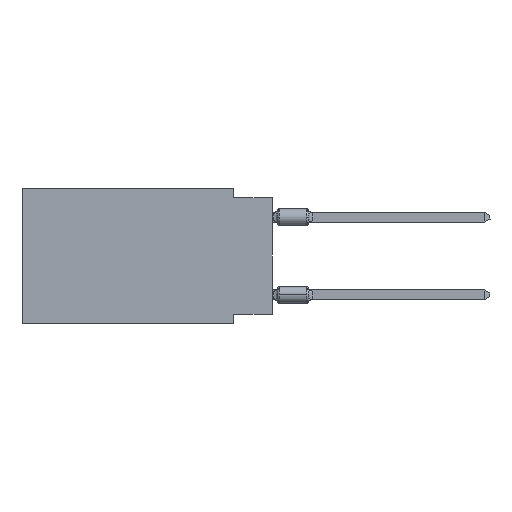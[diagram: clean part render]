
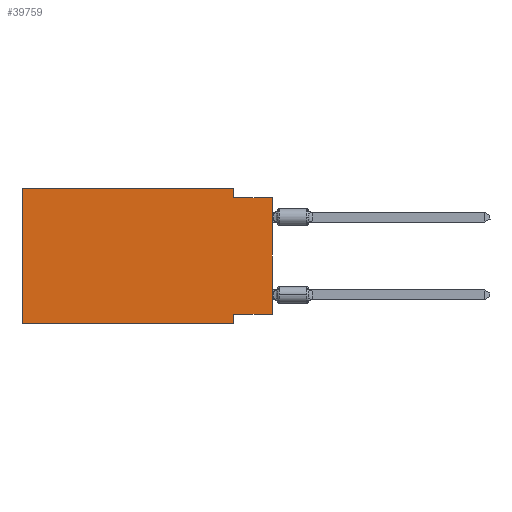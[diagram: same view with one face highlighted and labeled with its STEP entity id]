
A CAD part, left-side view. The second image highlights one B-rep face of the part: STEP entity #39759.
In plain terms, the highlighted planar face has unit normal (-1, 0, 0).
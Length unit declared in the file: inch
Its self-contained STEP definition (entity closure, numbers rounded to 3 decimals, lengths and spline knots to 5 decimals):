
#1094 = EDGE_CURVE ( 'NONE', #7200, #34271, #24321, .T. ) ;
#1792 = DIRECTION ( 'NONE',  ( 0., -1., 0. ) ) ;
#2064 = VECTOR ( 'NONE', #16429, 39.37008 ) ;
#2184 = DIRECTION ( 'NONE',  ( 0., 0., -1. ) ) ;
#2597 = DIRECTION ( 'NONE',  ( 0., 0., -1. ) ) ;
#3009 = VERTEX_POINT ( 'NONE', #53379 ) ;
#3027 = CARTESIAN_POINT ( 'NONE',  ( 0., 0.645, -0.35 ) ) ;
#5474 = CARTESIAN_POINT ( 'NONE',  ( 0., 0.1, -0.325 ) ) ;
#5514 = CARTESIAN_POINT ( 'NONE',  ( 0., 0.1, -0.025 ) ) ;
#6028 = CARTESIAN_POINT ( 'NONE',  ( 0., 0.645, 0. ) ) ;
#6404 = EDGE_CURVE ( 'NONE', #3009, #37174, #39988, .T. ) ;
#6475 = DIRECTION ( 'NONE',  ( 0., 1., 0. ) ) ;
#6872 = ORIENTED_EDGE ( 'NONE', *, *, #6404, .F. ) ;
#7200 = VERTEX_POINT ( 'NONE', #22787 ) ;
#7378 = EDGE_CURVE ( 'NONE', #37174, #37012, #45947, .T. ) ;
#9947 = LINE ( 'NONE', #36362, #50279 ) ;
#12422 = ORIENTED_EDGE ( 'NONE', *, *, #31131, .T. ) ;
#13573 = CARTESIAN_POINT ( 'NONE',  ( 0., 0.645, 0. ) ) ;
#15375 = AXIS2_PLACEMENT_3D ( 'NONE', #69291, #51464, #2597 ) ;
#16429 = DIRECTION ( 'NONE',  ( 0., 0., 1. ) ) ;
#19960 = DIRECTION ( 'NONE',  ( 0., -1., 0. ) ) ;
#20821 = ORIENTED_EDGE ( 'NONE', *, *, #7378, .F. ) ;
#22787 = CARTESIAN_POINT ( 'NONE',  ( 0., 0., -0.325 ) ) ;
#23121 = CARTESIAN_POINT ( 'NONE',  ( 0., 0.1, -0.35 ) ) ;
#23978 = CARTESIAN_POINT ( 'NONE',  ( 0., 0., -0.325 ) ) ;
#24211 = LINE ( 'NONE', #61638, #42753 ) ;
#24321 = LINE ( 'NONE', #23978, #45250 ) ;
#24451 = ORIENTED_EDGE ( 'NONE', *, *, #54711, .T. ) ;
#25794 = PLANE ( 'NONE',  #15375 ) ;
#27500 = DIRECTION ( 'NONE',  ( 0., 0., 1. ) ) ;
#27791 = CARTESIAN_POINT ( 'NONE',  ( 0., 0., -0.025 ) ) ;
#27834 = EDGE_CURVE ( 'NONE', #51029, #43485, #70277, .T. ) ;
#29914 = DIRECTION ( 'NONE',  ( 0., 0., -1. ) ) ;
#31131 = EDGE_CURVE ( 'NONE', #51029, #47694, #9947, .T. ) ;
#34271 = VERTEX_POINT ( 'NONE', #5474 ) ;
#36362 = CARTESIAN_POINT ( 'NONE',  ( 0., 0.645, -0.35 ) ) ;
#37012 = VERTEX_POINT ( 'NONE', #27791 ) ;
#37174 = VERTEX_POINT ( 'NONE', #5514 ) ;
#39305 = ORIENTED_EDGE ( 'NONE', *, *, #27834, .F. ) ;
#39759 = ADVANCED_FACE ( 'NONE', ( #52894 ), #25794, .F. ) ;
#39988 = LINE ( 'NONE', #55375, #59538 ) ;
#40474 = EDGE_CURVE ( 'NONE', #34271, #47694, #24211, .T. ) ;
#41664 = CARTESIAN_POINT ( 'NONE',  ( 0., 0., -0.025 ) ) ;
#42728 = EDGE_CURVE ( 'NONE', #43485, #3009, #62416, .T. ) ;
#42753 = VECTOR ( 'NONE', #29914, 39.37008 ) ;
#43485 = VERTEX_POINT ( 'NONE', #53410 ) ;
#45250 = VECTOR ( 'NONE', #6475, 39.37008 ) ;
#45718 = VECTOR ( 'NONE', #1792, 39.37008 ) ;
#45947 = LINE ( 'NONE', #41664, #47339 ) ;
#46823 = VECTOR ( 'NONE', #27500, 39.37008 ) ;
#47339 = VECTOR ( 'NONE', #68039, 39.37008 ) ;
#47694 = VERTEX_POINT ( 'NONE', #23121 ) ;
#50279 = VECTOR ( 'NONE', #19960, 39.37008 ) ;
#51029 = VERTEX_POINT ( 'NONE', #3027 ) ;
#51464 = DIRECTION ( 'NONE',  ( 1., 0., 0. ) ) ;
#52894 = FACE_OUTER_BOUND ( 'NONE', #61762, .T. ) ;
#53379 = CARTESIAN_POINT ( 'NONE',  ( 0., 0.1, 0. ) ) ;
#53410 = CARTESIAN_POINT ( 'NONE',  ( 0., 0.645, 0. ) ) ;
#54711 = EDGE_CURVE ( 'NONE', #7200, #37012, #65986, .T. ) ;
#54886 = ORIENTED_EDGE ( 'NONE', *, *, #1094, .F. ) ;
#55375 = CARTESIAN_POINT ( 'NONE',  ( 0., 0.1, 0. ) ) ;
#59538 = VECTOR ( 'NONE', #2184, 39.37008 ) ;
#59875 = ORIENTED_EDGE ( 'NONE', *, *, #40474, .F. ) ;
#61638 = CARTESIAN_POINT ( 'NONE',  ( 0., 0.1, -0.35 ) ) ;
#61762 = EDGE_LOOP ( 'NONE', ( #24451, #20821, #6872, #67454, #39305, #12422, #59875, #54886 ) ) ;
#62416 = LINE ( 'NONE', #13573, #45718 ) ;
#65986 = LINE ( 'NONE', #66675, #46823 ) ;
#66675 = CARTESIAN_POINT ( 'NONE',  ( 0., 0., 0. ) ) ;
#67454 = ORIENTED_EDGE ( 'NONE', *, *, #42728, .F. ) ;
#68039 = DIRECTION ( 'NONE',  ( 0., -1., 0. ) ) ;
#69291 = CARTESIAN_POINT ( 'NONE',  ( 0., 0.645, 0. ) ) ;
#70277 = LINE ( 'NONE', #6028, #2064 ) ;
